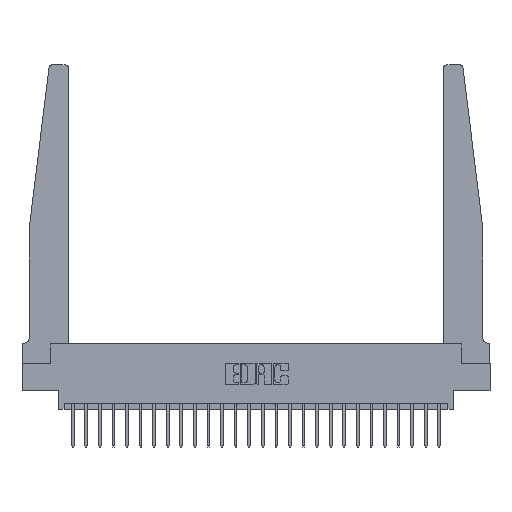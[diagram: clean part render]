
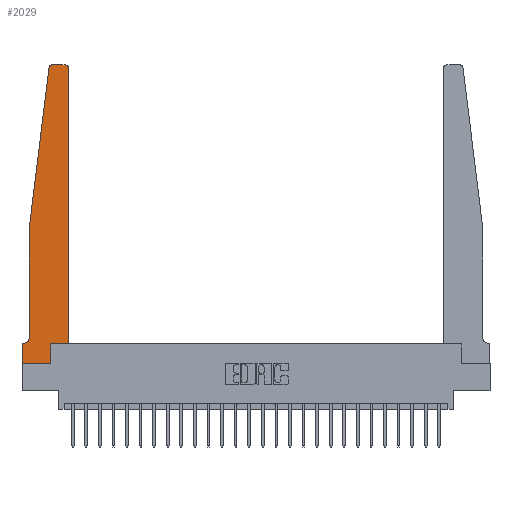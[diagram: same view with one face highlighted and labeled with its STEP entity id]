
A CAD part, top view. The second image highlights one B-rep face of the part: STEP entity #2029.
In plain terms, the highlighted planar face has unit normal (0, 0, 1).
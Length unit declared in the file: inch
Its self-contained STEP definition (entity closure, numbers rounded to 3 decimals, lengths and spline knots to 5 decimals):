
#91 = DIRECTION ( 'NONE',  ( 0., 1., 0. ) ) ;
#97 = EDGE_CURVE ( 'NONE', #8706, #12353, #1362, .T. ) ;
#406 = CARTESIAN_POINT ( 'NONE',  ( 0.2605, 0., 0.37 ) ) ;
#559 = LINE ( 'NONE', #8566, #8029 ) ;
#1045 = VECTOR ( 'NONE', #9952, 39.37008 ) ;
#1127 = CARTESIAN_POINT ( 'NONE',  ( 0.25, 2.75, 0.37 ) ) ;
#1314 = LINE ( 'NONE', #17007, #25079 ) ;
#1362 = LINE ( 'NONE', #19073, #3223 ) ;
#2029 = ADVANCED_FACE ( 'NONE', ( #11245 ), #20914, .T. ) ;
#2504 = ORIENTED_EDGE ( 'NONE', *, *, #18412, .T. ) ;
#2540 = EDGE_CURVE ( 'NONE', #12687, #7214, #18721, .T. ) ;
#2762 = CARTESIAN_POINT ( 'NONE',  ( 0.065, 0.1875, 0.37 ) ) ;
#2915 = EDGE_CURVE ( 'NONE', #5919, #12687, #15476, .T. ) ;
#3082 = CARTESIAN_POINT ( 'NONE',  ( 0.27653, 2.75, 0.37 ) ) ;
#3223 = VECTOR ( 'NONE', #22794, 39.37008 ) ;
#3309 = VERTEX_POINT ( 'NONE', #12345 ) ;
#3332 = EDGE_CURVE ( 'NONE', #18408, #5919, #559, .T. ) ;
#3586 = CARTESIAN_POINT ( 'NONE',  ( 0.2605, 0.18, 0.37 ) ) ;
#3809 = DIRECTION ( 'NONE',  ( -1., 0., 0. ) ) ;
#3964 = LINE ( 'NONE', #3586, #17792 ) ;
#4011 = VECTOR ( 'NONE', #8457, 39.37008 ) ;
#4162 = EDGE_CURVE ( 'NONE', #25238, #24867, #22415, .T. ) ;
#4390 = CARTESIAN_POINT ( 'NONE',  ( 0.425, 2.72, 0.37 ) ) ;
#4703 = DIRECTION ( 'NONE',  ( 0., 0., 1. ) ) ;
#4970 = DIRECTION ( 'NONE',  ( 0., 0., 1. ) ) ;
#5036 = ORIENTED_EDGE ( 'NONE', *, *, #4162, .T. ) ;
#5122 = AXIS2_PLACEMENT_3D ( 'NONE', #21499, #25247, #3809 ) ;
#5457 = LINE ( 'NONE', #23539, #24237 ) ;
#5833 = DIRECTION ( 'NONE',  ( 1., 0., 0. ) ) ;
#5919 = VERTEX_POINT ( 'NONE', #4390 ) ;
#7165 = CARTESIAN_POINT ( 'NONE',  ( 0.24675, 2.72367, 0.37 ) ) ;
#7214 = VERTEX_POINT ( 'NONE', #3082 ) ;
#7781 = EDGE_LOOP ( 'NONE', ( #24630, #23535, #5036, #12935, #18615, #22153, #24628, #8819, #13310, #2504, #10576, #25396 ) ) ;
#8029 = VECTOR ( 'NONE', #17919, 39.37008 ) ;
#8457 = DIRECTION ( 'NONE',  ( -1., 0., 0. ) ) ;
#8566 = CARTESIAN_POINT ( 'NONE',  ( 0.425, 0.18, 0.37 ) ) ;
#8644 = CARTESIAN_POINT ( 'NONE',  ( 0.065, 1.25, 0.37 ) ) ;
#8706 = VERTEX_POINT ( 'NONE', #14221 ) ;
#8819 = ORIENTED_EDGE ( 'NONE', *, *, #24593, .T. ) ;
#8995 = DIRECTION ( 'NONE',  ( -1., 0., 0. ) ) ;
#9617 = CARTESIAN_POINT ( 'NONE',  ( 0.065, 0.2375, 0.37 ) ) ;
#9952 = DIRECTION ( 'NONE',  ( 0., -1., 0. ) ) ;
#10465 = LINE ( 'NONE', #18371, #1045 ) ;
#10576 = ORIENTED_EDGE ( 'NONE', *, *, #3332, .T. ) ;
#10791 = DIRECTION ( 'NONE',  ( 1., 0., 0. ) ) ;
#11065 = CARTESIAN_POINT ( 'NONE',  ( 0.27653, 2.72, 0.37 ) ) ;
#11245 = FACE_OUTER_BOUND ( 'NONE', #7781, .T. ) ;
#11366 = CARTESIAN_POINT ( 'NONE',  ( 0., 0.1875, 0.37 ) ) ;
#11493 = DIRECTION ( 'NONE',  ( 0., 0., 1. ) ) ;
#11741 = AXIS2_PLACEMENT_3D ( 'NONE', #18068, #4703, #24100 ) ;
#11885 = VERTEX_POINT ( 'NONE', #406 ) ;
#12345 = CARTESIAN_POINT ( 'NONE',  ( 0.015, 0.1875, 0.37 ) ) ;
#12353 = VERTEX_POINT ( 'NONE', #18611 ) ;
#12551 = VECTOR ( 'NONE', #8995, 39.37008 ) ;
#12687 = VERTEX_POINT ( 'NONE', #24243 ) ;
#12732 = LINE ( 'NONE', #2762, #4011 ) ;
#12875 = EDGE_CURVE ( 'NONE', #7214, #25238, #13050, .T. ) ;
#12935 = ORIENTED_EDGE ( 'NONE', *, *, #20340, .T. ) ;
#13050 = CIRCLE ( 'NONE', #21686, 0.03 ) ;
#13310 = ORIENTED_EDGE ( 'NONE', *, *, #16538, .T. ) ;
#14221 = CARTESIAN_POINT ( 'NONE',  ( 0., 0.1875, 0.37 ) ) ;
#14263 = AXIS2_PLACEMENT_3D ( 'NONE', #11366, #11493, #21041 ) ;
#15476 = CIRCLE ( 'NONE', #11741, 0.03 ) ;
#15577 = CARTESIAN_POINT ( 'NONE',  ( 0.2605, 0.18, 0.37 ) ) ;
#15590 = EDGE_CURVE ( 'NONE', #16928, #3309, #24110, .T. ) ;
#16538 = EDGE_CURVE ( 'NONE', #11885, #18353, #3964, .T. ) ;
#16665 = DIRECTION ( 'NONE',  ( -0.122, -0.992, 0. ) ) ;
#16928 = VERTEX_POINT ( 'NONE', #9617 ) ;
#17007 = CARTESIAN_POINT ( 'NONE',  ( 0., 0., 0.37 ) ) ;
#17792 = VECTOR ( 'NONE', #91, 39.37008 ) ;
#17919 = DIRECTION ( 'NONE',  ( 0., 1., 0. ) ) ;
#18068 = CARTESIAN_POINT ( 'NONE',  ( 0.395, 2.72, 0.37 ) ) ;
#18353 = VERTEX_POINT ( 'NONE', #15577 ) ;
#18371 = CARTESIAN_POINT ( 'NONE',  ( 0.065, 1.25, 0.37 ) ) ;
#18408 = VERTEX_POINT ( 'NONE', #19169 ) ;
#18412 = EDGE_CURVE ( 'NONE', #18353, #18408, #5457, .T. ) ;
#18611 = CARTESIAN_POINT ( 'NONE',  ( 0., 0., 0.37 ) ) ;
#18615 = ORIENTED_EDGE ( 'NONE', *, *, #15590, .T. ) ;
#18721 = LINE ( 'NONE', #1127, #12551 ) ;
#19073 = CARTESIAN_POINT ( 'NONE',  ( 0., 0., 0.37 ) ) ;
#19169 = CARTESIAN_POINT ( 'NONE',  ( 0.425, 0.18, 0.37 ) ) ;
#19216 = VECTOR ( 'NONE', #16665, 39.37008 ) ;
#20340 = EDGE_CURVE ( 'NONE', #24867, #16928, #10465, .T. ) ;
#20914 = PLANE ( 'NONE',  #14263 ) ;
#21041 = DIRECTION ( 'NONE',  ( 1., 0., 0. ) ) ;
#21324 = DIRECTION ( 'NONE',  ( 1., 0., 0. ) ) ;
#21499 = CARTESIAN_POINT ( 'NONE',  ( 0.015, 0.2375, 0.37 ) ) ;
#21686 = AXIS2_PLACEMENT_3D ( 'NONE', #11065, #4970, #10791 ) ;
#22153 = ORIENTED_EDGE ( 'NONE', *, *, #24015, .T. ) ;
#22415 = LINE ( 'NONE', #22537, #19216 ) ;
#22537 = CARTESIAN_POINT ( 'NONE',  ( 0.065, 1.25, 0.37 ) ) ;
#22794 = DIRECTION ( 'NONE',  ( 0., -1., 0. ) ) ;
#23535 = ORIENTED_EDGE ( 'NONE', *, *, #12875, .T. ) ;
#23539 = CARTESIAN_POINT ( 'NONE',  ( 0.425, 0.18, 0.37 ) ) ;
#24015 = EDGE_CURVE ( 'NONE', #3309, #8706, #12732, .T. ) ;
#24100 = DIRECTION ( 'NONE',  ( 1., 0., 0. ) ) ;
#24110 = CIRCLE ( 'NONE', #5122, 0.05 ) ;
#24237 = VECTOR ( 'NONE', #5833, 39.37008 ) ;
#24243 = CARTESIAN_POINT ( 'NONE',  ( 0.395, 2.75, 0.37 ) ) ;
#24593 = EDGE_CURVE ( 'NONE', #12353, #11885, #1314, .T. ) ;
#24628 = ORIENTED_EDGE ( 'NONE', *, *, #97, .T. ) ;
#24630 = ORIENTED_EDGE ( 'NONE', *, *, #2540, .T. ) ;
#24867 = VERTEX_POINT ( 'NONE', #8644 ) ;
#25079 = VECTOR ( 'NONE', #21324, 39.37008 ) ;
#25238 = VERTEX_POINT ( 'NONE', #7165 ) ;
#25247 = DIRECTION ( 'NONE',  ( 0., 0., -1. ) ) ;
#25396 = ORIENTED_EDGE ( 'NONE', *, *, #2915, .T. ) ;
